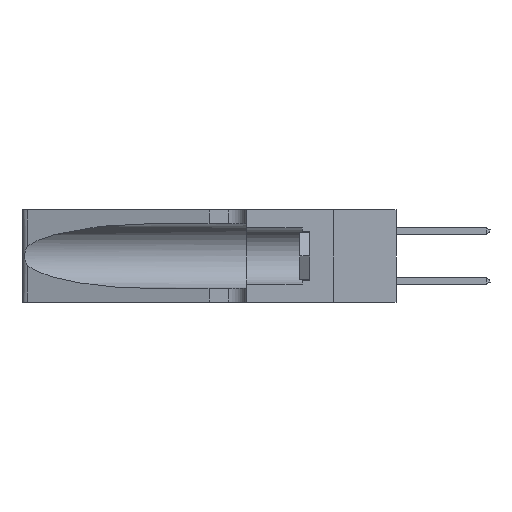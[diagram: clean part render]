
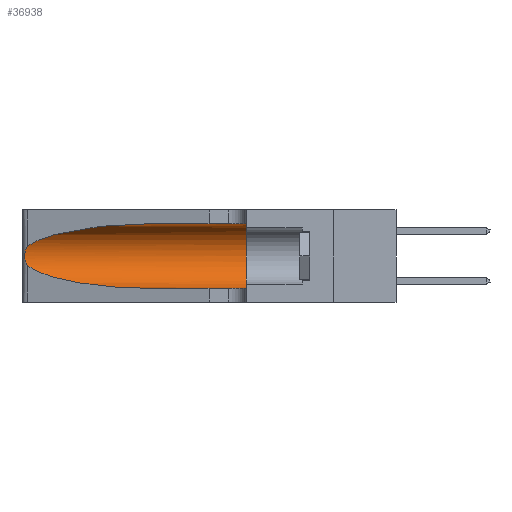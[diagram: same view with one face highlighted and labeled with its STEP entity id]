
A CAD part, left-side view. The second image highlights one B-rep face of the part: STEP entity #36938.
In plain terms, the highlighted cylindrical face has radius 3.308 mm (diameter 6.617 mm), a partial arc.
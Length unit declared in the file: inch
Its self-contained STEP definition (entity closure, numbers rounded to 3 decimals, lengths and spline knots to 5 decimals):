
#152 = CARTESIAN_POINT ( 'NONE',  ( 0.1305, 0.35, 0.185 ) ) ;
#267 = VERTEX_POINT ( 'NONE', #27237 ) ;
#707 = CARTESIAN_POINT ( 'NONE',  ( 0.26075, 1.23896, 0.19203 ) ) ;
#1458 = CARTESIAN_POINT ( 'NONE',  ( 0.1305, 0.72297, 0.05475 ) ) ;
#2678 = VECTOR ( 'NONE', #11497, 39.37008 ) ;
#3155 = CARTESIAN_POINT ( 'NONE',  ( 0.1305, 1.61858, 0.31525 ) ) ;
#3227 = DIRECTION ( 'NONE',  ( 0., 0., 1. ) ) ;
#3759 = CARTESIAN_POINT ( 'NONE',  ( 0.26017, 1.23833, 0.17102 ) ) ;
#4601 = CARTESIAN_POINT ( 'NONE',  ( 0.25487, 1.22718, 0.22369 ) ) ;
#5141 = EDGE_CURVE ( 'NONE', #33676, #23514, #15698, .T. ) ;
#5337 = ORIENTED_EDGE ( 'NONE', *, *, #32920, .T. ) ;
#6393 = CARTESIAN_POINT ( 'NONE',  ( 0.18966, 0.96281, 0.31525 ) ) ;
#6808 = CARTESIAN_POINT ( 'NONE',  ( 0.25789, 1.23486, 0.15765 ) ) ;
#7114 = AXIS2_PLACEMENT_3D ( 'NONE', #152, #21296, #3227 ) ;
#7426 = CARTESIAN_POINT ( 'NONE',  ( 0.2373, 1.15595, 0.08982 ) ) ;
#7974 = VERTEX_POINT ( 'NONE', #9106 ) ;
#8005 = EDGE_CURVE ( 'NONE', #267, #34350, #35279, .T. ) ;
#8185 =( BOUNDED_CURVE ( )  B_SPLINE_CURVE ( 3, ( #22430, #7426, #19555, #1458 ),
 .UNSPECIFIED., .F., .F. ) 
 B_SPLINE_CURVE_WITH_KNOTS ( ( 4, 4 ),
 ( 3.44316, 4.71239 ),
 .UNSPECIFIED. ) 
 CURVE ( )  GEOMETRIC_REPRESENTATION_ITEM ( )  RATIONAL_B_SPLINE_CURVE ( ( 1., 0.87, 0.87, 1. ) ) 
 REPRESENTATION_ITEM ( '' )  );
#9106 = CARTESIAN_POINT ( 'NONE',  ( 0.1305, 0.72297, 0.05475 ) ) ;
#9484 = CARTESIAN_POINT ( 'NONE',  ( 0.25487, 1.22718, 0.22369 ) ) ;
#9765 = CARTESIAN_POINT ( 'NONE',  ( 0.25487, 1.22718, 0.22369 ) ) ;
#9840 = CYLINDRICAL_SURFACE ( 'NONE', #34730, 0.13025 ) ;
#9894 = CARTESIAN_POINT ( 'NONE',  ( 0.25555, 1.22993, 0.14849 ) ) ;
#10406 = B_SPLINE_CURVE_WITH_KNOTS ( 'NONE', 3,
 ( #9765, #12774, #33800, #15795, #36805, #18816, #707, #21827, #3759, #24861, #6808, #27895, #9894, #30924 ),
 .UNSPECIFIED., .F., .F.,
 ( 4, 2, 2, 2, 2, 2, 4 ),
 ( 0., 0.00027, 0.00053, 0.00107, 0.0016, 0.00187, 0.00214 ),
 .UNSPECIFIED. ) ;
#10751 = LINE ( 'NONE', #29558, #2678 ) ;
#10773 = FACE_OUTER_BOUND ( 'NONE', #28660, .T. ) ;
#10963 = CARTESIAN_POINT ( 'NONE',  ( 0.1305, 0.72297, 0.31525 ) ) ;
#11497 = DIRECTION ( 'NONE',  ( 0., -1., 0. ) ) ;
#12774 = CARTESIAN_POINT ( 'NONE',  ( 0.25555, 1.22994, 0.2215 ) ) ;
#13045 = CARTESIAN_POINT ( 'NONE',  ( 0.1305, 1.61858, 0.185 ) ) ;
#15698 =( BOUNDED_CURVE ( )  B_SPLINE_CURVE ( 3, ( #27502, #6393, #27364, #9484 ),
 .UNSPECIFIED., .F., .F. ) 
 B_SPLINE_CURVE_WITH_KNOTS ( ( 4, 4 ),
 ( 1.5708, 2.84003 ),
 .UNSPECIFIED. ) 
 CURVE ( )  GEOMETRIC_REPRESENTATION_ITEM ( )  RATIONAL_B_SPLINE_CURVE ( ( 1., 0.87, 0.87, 1. ) ) 
 REPRESENTATION_ITEM ( '' )  );
#15795 = CARTESIAN_POINT ( 'NONE',  ( 0.25787, 1.23484, 0.2124 ) ) ;
#16074 = DIRECTION ( 'NONE',  ( 0., -1., 0. ) ) ;
#16280 = EDGE_CURVE ( 'NONE', #23514, #30757, #10406, .T. ) ;
#18816 = CARTESIAN_POINT ( 'NONE',  ( 0.26018, 1.23835, 0.19895 ) ) ;
#19555 = CARTESIAN_POINT ( 'NONE',  ( 0.18966, 0.96281, 0.05475 ) ) ;
#20068 = EDGE_CURVE ( 'NONE', #33676, #267, #23347, .T. ) ;
#21296 = DIRECTION ( 'NONE',  ( 0., 1., 0. ) ) ;
#21827 = CARTESIAN_POINT ( 'NONE',  ( 0.26075, 1.23896, 0.178 ) ) ;
#22430 = CARTESIAN_POINT ( 'NONE',  ( 0.25487, 1.22718, 0.14631 ) ) ;
#23347 = LINE ( 'NONE', #3155, #37446 ) ;
#23514 = VERTEX_POINT ( 'NONE', #4601 ) ;
#24861 = CARTESIAN_POINT ( 'NONE',  ( 0.25856, 1.23593, 0.16098 ) ) ;
#25602 = EDGE_CURVE ( 'NONE', #7974, #34350, #10751, .T. ) ;
#26371 = ORIENTED_EDGE ( 'NONE', *, *, #8005, .F. ) ;
#26432 = CARTESIAN_POINT ( 'NONE',  ( 0.1305, 0.35, 0.05475 ) ) ;
#27237 = CARTESIAN_POINT ( 'NONE',  ( 0.1305, 0.35, 0.31525 ) ) ;
#27364 = CARTESIAN_POINT ( 'NONE',  ( 0.2373, 1.15595, 0.28018 ) ) ;
#27502 = CARTESIAN_POINT ( 'NONE',  ( 0.1305, 0.72297, 0.31525 ) ) ;
#27895 = CARTESIAN_POINT ( 'NONE',  ( 0.25639, 1.23186, 0.15144 ) ) ;
#28660 = EDGE_LOOP ( 'NONE', ( #29090, #31048, #5337, #29055, #26371, #35359 ) ) ;
#29055 = ORIENTED_EDGE ( 'NONE', *, *, #25602, .T. ) ;
#29090 = ORIENTED_EDGE ( 'NONE', *, *, #5141, .T. ) ;
#29558 = CARTESIAN_POINT ( 'NONE',  ( 0.1305, 1.61858, 0.05475 ) ) ;
#30757 = VERTEX_POINT ( 'NONE', #35037 ) ;
#30924 = CARTESIAN_POINT ( 'NONE',  ( 0.25487, 1.22718, 0.14631 ) ) ;
#31048 = ORIENTED_EDGE ( 'NONE', *, *, #16280, .T. ) ;
#32920 = EDGE_CURVE ( 'NONE', #30757, #7974, #8185, .T. ) ;
#33335 = DIRECTION ( 'NONE',  ( 0., -1., 0. ) ) ;
#33676 = VERTEX_POINT ( 'NONE', #10963 ) ;
#33800 = CARTESIAN_POINT ( 'NONE',  ( 0.25639, 1.23184, 0.21858 ) ) ;
#34350 = VERTEX_POINT ( 'NONE', #26432 ) ;
#34730 = AXIS2_PLACEMENT_3D ( 'NONE', #13045, #16074, #37079 ) ;
#35037 = CARTESIAN_POINT ( 'NONE',  ( 0.25487, 1.22718, 0.14631 ) ) ;
#35279 = CIRCLE ( 'NONE', #7114, 0.13025 ) ;
#35359 = ORIENTED_EDGE ( 'NONE', *, *, #20068, .F. ) ;
#36805 = CARTESIAN_POINT ( 'NONE',  ( 0.25854, 1.2359, 0.20912 ) ) ;
#36938 = ADVANCED_FACE ( 'NONE', ( #10773 ), #9840, .F. ) ;
#37079 = DIRECTION ( 'NONE',  ( 0., 0., -1. ) ) ;
#37446 = VECTOR ( 'NONE', #33335, 39.37008 ) ;
